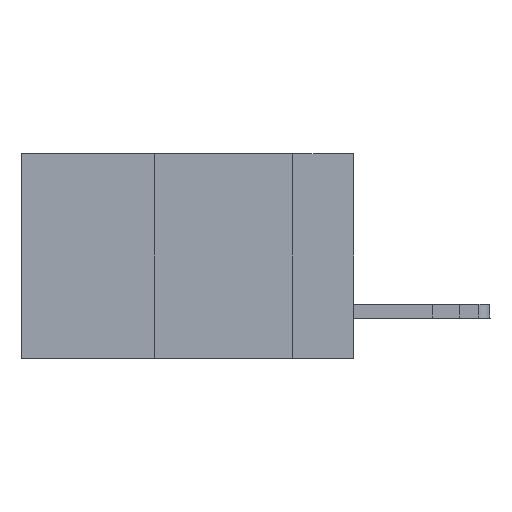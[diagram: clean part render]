
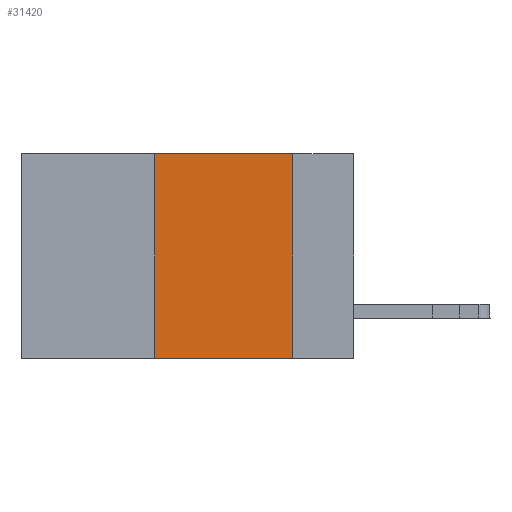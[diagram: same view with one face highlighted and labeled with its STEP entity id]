
A CAD part, left-side view. The second image highlights one B-rep face of the part: STEP entity #31420.
In plain terms, the highlighted planar face has unit normal (-1, 0, 0).
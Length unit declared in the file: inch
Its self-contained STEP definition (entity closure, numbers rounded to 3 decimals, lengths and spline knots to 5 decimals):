
#3107 = VERTEX_POINT ( 'NONE', #25744 ) ;
#4827 = CARTESIAN_POINT ( 'NONE',  ( 0., 0.6, 0. ) ) ;
#5057 = VECTOR ( 'NONE', #10746, 39.37008 ) ;
#5154 = CARTESIAN_POINT ( 'NONE',  ( 0., 0.36, -0.37 ) ) ;
#6258 = LINE ( 'NONE', #19080, #12106 ) ;
#7310 = DIRECTION ( 'NONE',  ( 0., 0., -1. ) ) ;
#8289 = CARTESIAN_POINT ( 'NONE',  ( 0., 0.36, 0. ) ) ;
#8474 = DIRECTION ( 'NONE',  ( 0., -1., 0. ) ) ;
#8549 = VECTOR ( 'NONE', #18263, 39.37008 ) ;
#10746 = DIRECTION ( 'NONE',  ( 0., -1., 0. ) ) ;
#11056 = ORIENTED_EDGE ( 'NONE', *, *, #20858, .F. ) ;
#11769 = VECTOR ( 'NONE', #8474, 39.37008 ) ;
#12106 = VECTOR ( 'NONE', #21457, 39.37008 ) ;
#13825 = CARTESIAN_POINT ( 'NONE',  ( 0., 0.11, -0.37 ) ) ;
#13876 = AXIS2_PLACEMENT_3D ( 'NONE', #4827, #22321, #7310 ) ;
#13992 = EDGE_CURVE ( 'NONE', #17737, #24572, #18396, .T. ) ;
#14022 = FACE_OUTER_BOUND ( 'NONE', #31777, .T. ) ;
#15599 = CARTESIAN_POINT ( 'NONE',  ( 0., 0.36, 0. ) ) ;
#17737 = VERTEX_POINT ( 'NONE', #5154 ) ;
#18263 = DIRECTION ( 'NONE',  ( 0., 0., 1. ) ) ;
#18355 = CARTESIAN_POINT ( 'NONE',  ( 0., 0.6, -0.37 ) ) ;
#18396 = LINE ( 'NONE', #18355, #11769 ) ;
#19080 = CARTESIAN_POINT ( 'NONE',  ( 0., 0.11, 0. ) ) ;
#19751 = PLANE ( 'NONE',  #13876 ) ;
#20858 = EDGE_CURVE ( 'NONE', #17737, #26136, #28444, .T. ) ;
#21457 = DIRECTION ( 'NONE',  ( 0., 0., -1. ) ) ;
#22321 = DIRECTION ( 'NONE',  ( 1., 0., 0. ) ) ;
#23213 = CARTESIAN_POINT ( 'NONE',  ( 0., 0.6, 0. ) ) ;
#23860 = EDGE_CURVE ( 'NONE', #26136, #3107, #30805, .T. ) ;
#24572 = VERTEX_POINT ( 'NONE', #13825 ) ;
#25744 = CARTESIAN_POINT ( 'NONE',  ( 0., 0.11, 0. ) ) ;
#26136 = VERTEX_POINT ( 'NONE', #8289 ) ;
#26691 = ORIENTED_EDGE ( 'NONE', *, *, #31276, .F. ) ;
#28444 = LINE ( 'NONE', #15599, #8549 ) ;
#30185 = ORIENTED_EDGE ( 'NONE', *, *, #13992, .T. ) ;
#30805 = LINE ( 'NONE', #23213, #5057 ) ;
#31276 = EDGE_CURVE ( 'NONE', #3107, #24572, #6258, .T. ) ;
#31319 = ORIENTED_EDGE ( 'NONE', *, *, #23860, .F. ) ;
#31420 = ADVANCED_FACE ( 'NONE', ( #14022 ), #19751, .F. ) ;
#31777 = EDGE_LOOP ( 'NONE', ( #26691, #31319, #11056, #30185 ) ) ;
